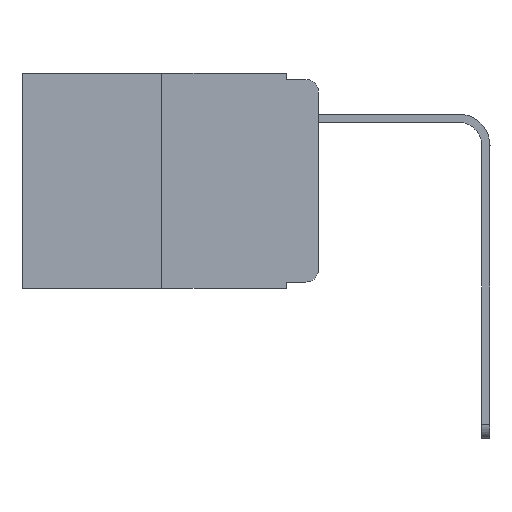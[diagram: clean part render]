
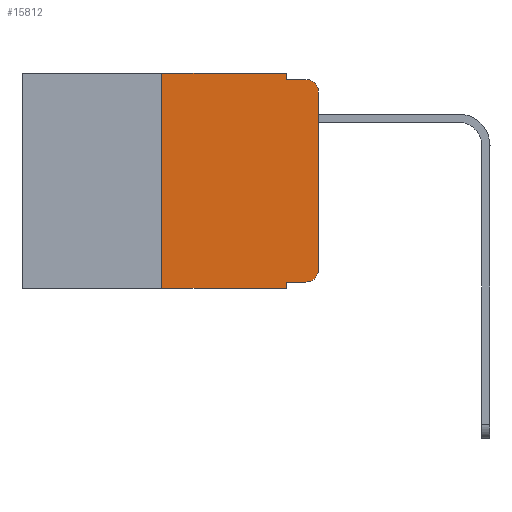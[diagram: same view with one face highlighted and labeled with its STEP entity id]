
A CAD part, left-side view. The second image highlights one B-rep face of the part: STEP entity #15812.
In plain terms, the highlighted planar face has unit normal (-1, 0, 0).
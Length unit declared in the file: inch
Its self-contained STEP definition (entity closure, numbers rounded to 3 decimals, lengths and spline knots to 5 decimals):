
#72 = EDGE_CURVE ( 'NONE', #14348, #3779, #12541, .T. ) ;
#226 = DIRECTION ( 'NONE',  ( 0., 0., 1. ) ) ;
#395 = CARTESIAN_POINT ( 'NONE',  ( 0., 0.051, 0. ) ) ;
#409 = EDGE_CURVE ( 'NONE', #2820, #8085, #8511, .T. ) ;
#560 = CARTESIAN_POINT ( 'NONE',  ( 0., 0.25, 0. ) ) ;
#724 = ORIENTED_EDGE ( 'NONE', *, *, #9500, .F. ) ;
#970 = LINE ( 'NONE', #13414, #4964 ) ;
#1144 = VECTOR ( 'NONE', #6472, 39.37008 ) ;
#1381 = CARTESIAN_POINT ( 'NONE',  ( 0., 0.051, -0.01 ) ) ;
#1577 = CARTESIAN_POINT ( 'NONE',  ( 0., 0.051, -0.01 ) ) ;
#1872 = VERTEX_POINT ( 'NONE', #12797 ) ;
#2077 = ORIENTED_EDGE ( 'NONE', *, *, #8630, .F. ) ;
#2474 = EDGE_CURVE ( 'NONE', #1872, #14348, #15052, .T. ) ;
#2820 = VERTEX_POINT ( 'NONE', #4243 ) ;
#3147 = ORIENTED_EDGE ( 'NONE', *, *, #13919, .T. ) ;
#3193 = EDGE_LOOP ( 'NONE', ( #12736, #3147, #2077, #17071, #724, #5308, #9417, #4608, #8288, #15742 ) ) ;
#3779 = VERTEX_POINT ( 'NONE', #11628 ) ;
#3955 = DIRECTION ( 'NONE',  ( 0., -1., 0. ) ) ;
#4243 = CARTESIAN_POINT ( 'NONE',  ( 0., 0.25, -0.343 ) ) ;
#4278 = VECTOR ( 'NONE', #8474, 39.37008 ) ;
#4290 = CARTESIAN_POINT ( 'NONE',  ( 0., 0.051, 0. ) ) ;
#4396 = DIRECTION ( 'NONE',  ( -1., 0., 0. ) ) ;
#4568 = CARTESIAN_POINT ( 'NONE',  ( 0., 0.02, -0.03 ) ) ;
#4608 = ORIENTED_EDGE ( 'NONE', *, *, #16324, .F. ) ;
#4964 = VECTOR ( 'NONE', #16137, 39.37008 ) ;
#4978 = VERTEX_POINT ( 'NONE', #395 ) ;
#5035 = DIRECTION ( 'NONE',  ( 0., 0., -1. ) ) ;
#5197 = CARTESIAN_POINT ( 'NONE',  ( 0., 0.051, -0.343 ) ) ;
#5221 = VERTEX_POINT ( 'NONE', #5197 ) ;
#5308 = ORIENTED_EDGE ( 'NONE', *, *, #409, .F. ) ;
#5373 = CARTESIAN_POINT ( 'NONE',  ( 0., 0.02, -0.333 ) ) ;
#5418 = VECTOR ( 'NONE', #5675, 39.37008 ) ;
#5515 = LINE ( 'NONE', #6567, #15891 ) ;
#5522 = VERTEX_POINT ( 'NONE', #6110 ) ;
#5675 = DIRECTION ( 'NONE',  ( 0., 0., -1. ) ) ;
#5794 = DIRECTION ( 'NONE',  ( 0., 0., -1. ) ) ;
#6110 = CARTESIAN_POINT ( 'NONE',  ( 0., 0.02, -0.01 ) ) ;
#6265 = VERTEX_POINT ( 'NONE', #1381 ) ;
#6472 = DIRECTION ( 'NONE',  ( 0., 0., 1. ) ) ;
#6567 = CARTESIAN_POINT ( 'NONE',  ( 0., 0.473, -0.343 ) ) ;
#6710 = AXIS2_PLACEMENT_3D ( 'NONE', #16325, #6961, #13756 ) ;
#6961 = DIRECTION ( 'NONE',  ( 1., 0., 0. ) ) ;
#6999 = LINE ( 'NONE', #1577, #4278 ) ;
#7335 = LINE ( 'NONE', #4290, #5418 ) ;
#7454 = VECTOR ( 'NONE', #17049, 39.37008 ) ;
#7574 = DIRECTION ( 'NONE',  ( -1., 0., 0. ) ) ;
#8056 = CARTESIAN_POINT ( 'NONE',  ( 0., 0.473, 0. ) ) ;
#8085 = VERTEX_POINT ( 'NONE', #560 ) ;
#8147 = VECTOR ( 'NONE', #226, 39.37008 ) ;
#8288 = ORIENTED_EDGE ( 'NONE', *, *, #2474, .T. ) ;
#8397 = PLANE ( 'NONE',  #6710 ) ;
#8474 = DIRECTION ( 'NONE',  ( 0., -1., 0. ) ) ;
#8511 = LINE ( 'NONE', #9250, #1144 ) ;
#8630 = EDGE_CURVE ( 'NONE', #6265, #5522, #6999, .T. ) ;
#9057 = EDGE_CURVE ( 'NONE', #2820, #5221, #5515, .T. ) ;
#9250 = CARTESIAN_POINT ( 'NONE',  ( 0., 0.25, 0. ) ) ;
#9417 = ORIENTED_EDGE ( 'NONE', *, *, #9057, .T. ) ;
#9500 = EDGE_CURVE ( 'NONE', #8085, #4978, #15651, .T. ) ;
#10504 = CIRCLE ( 'NONE', #14508, 0.02 ) ;
#10666 = FACE_OUTER_BOUND ( 'NONE', #3193, .T. ) ;
#10848 = CARTESIAN_POINT ( 'NONE',  ( 0., 0., 0. ) ) ;
#11433 = EDGE_CURVE ( 'NONE', #4978, #6265, #7335, .T. ) ;
#11628 = CARTESIAN_POINT ( 'NONE',  ( 0., 0., -0.313 ) ) ;
#11860 = VERTEX_POINT ( 'NONE', #13911 ) ;
#12243 = VECTOR ( 'NONE', #3955, 39.37008 ) ;
#12541 = CIRCLE ( 'NONE', #13702, 0.02 ) ;
#12736 = ORIENTED_EDGE ( 'NONE', *, *, #15175, .T. ) ;
#12797 = CARTESIAN_POINT ( 'NONE',  ( 0., 0.051, -0.333 ) ) ;
#13120 = CARTESIAN_POINT ( 'NONE',  ( 0., 0.02, -0.313 ) ) ;
#13414 = CARTESIAN_POINT ( 'NONE',  ( 0., 0.051, 0. ) ) ;
#13702 = AXIS2_PLACEMENT_3D ( 'NONE', #13120, #7574, #5035 ) ;
#13756 = DIRECTION ( 'NONE',  ( 0., 0., -1. ) ) ;
#13911 = CARTESIAN_POINT ( 'NONE',  ( 0., 0., -0.03 ) ) ;
#13919 = EDGE_CURVE ( 'NONE', #11860, #5522, #10504, .T. ) ;
#14348 = VERTEX_POINT ( 'NONE', #5373 ) ;
#14508 = AXIS2_PLACEMENT_3D ( 'NONE', #4568, #4396, #5794 ) ;
#14776 = DIRECTION ( 'NONE',  ( 0., -1., 0. ) ) ;
#15052 = LINE ( 'NONE', #16860, #7454 ) ;
#15175 = EDGE_CURVE ( 'NONE', #3779, #11860, #16616, .T. ) ;
#15651 = LINE ( 'NONE', #8056, #12243 ) ;
#15742 = ORIENTED_EDGE ( 'NONE', *, *, #72, .T. ) ;
#15812 = ADVANCED_FACE ( 'NONE', ( #10666 ), #8397, .F. ) ;
#15891 = VECTOR ( 'NONE', #14776, 39.37008 ) ;
#16137 = DIRECTION ( 'NONE',  ( 0., 0., -1. ) ) ;
#16324 = EDGE_CURVE ( 'NONE', #1872, #5221, #970, .T. ) ;
#16325 = CARTESIAN_POINT ( 'NONE',  ( 0., 0.473, 0. ) ) ;
#16616 = LINE ( 'NONE', #10848, #8147 ) ;
#16860 = CARTESIAN_POINT ( 'NONE',  ( 0., 0.051, -0.333 ) ) ;
#17049 = DIRECTION ( 'NONE',  ( 0., -1., 0. ) ) ;
#17071 = ORIENTED_EDGE ( 'NONE', *, *, #11433, .F. ) ;
